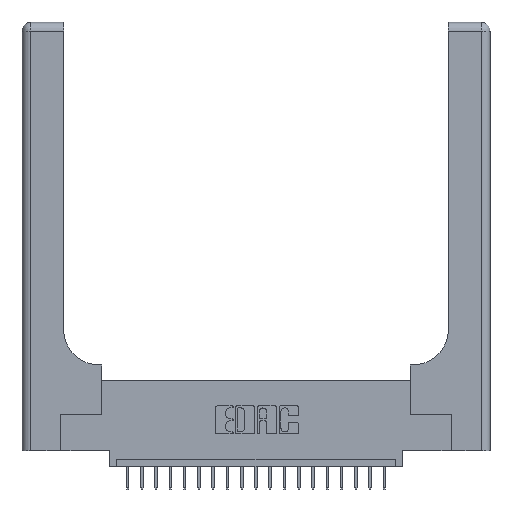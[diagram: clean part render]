
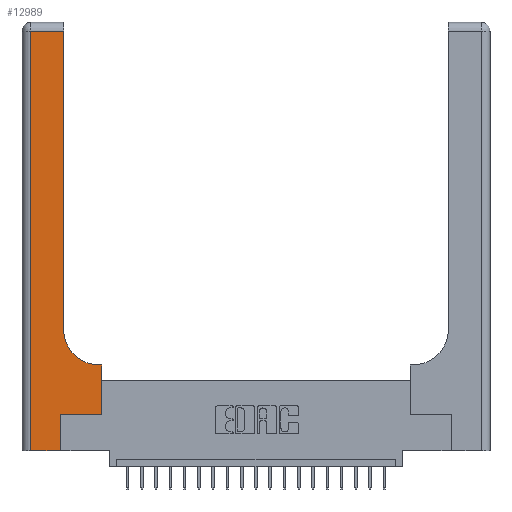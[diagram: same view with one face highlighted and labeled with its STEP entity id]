
A CAD part, top view. The second image highlights one B-rep face of the part: STEP entity #12989.
In plain terms, the highlighted planar face has unit normal (0, 0, 1).
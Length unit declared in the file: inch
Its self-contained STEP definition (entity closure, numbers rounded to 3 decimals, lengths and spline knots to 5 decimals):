
#396 = CARTESIAN_POINT ( 'NONE',  ( 0., 2.94, 0.37 ) ) ;
#868 = EDGE_CURVE ( 'NONE', #4343, #5429, #11607, .T. ) ;
#970 = CARTESIAN_POINT ( 'NONE',  ( 0.269, 0., 0.37 ) ) ;
#1243 = VERTEX_POINT ( 'NONE', #14700 ) ;
#1322 = CARTESIAN_POINT ( 'NONE',  ( 0.2915, 0.85, 0.37 ) ) ;
#1412 = DIRECTION ( 'NONE',  ( 1., 0., 0. ) ) ;
#2134 = DIRECTION ( 'NONE',  ( -1., 0., 0. ) ) ;
#2231 = CARTESIAN_POINT ( 'NONE',  ( 0.2915, 0.6, 0.37 ) ) ;
#2560 = EDGE_CURVE ( 'NONE', #10002, #20241, #6336, .T. ) ;
#2921 = ORIENTED_EDGE ( 'NONE', *, *, #21760, .T. ) ;
#3001 = EDGE_CURVE ( 'NONE', #5429, #19911, #18984, .T. ) ;
#3715 = DIRECTION ( 'NONE',  ( 0., 1., 0. ) ) ;
#4217 = ORIENTED_EDGE ( 'NONE', *, *, #19364, .T. ) ;
#4343 = VERTEX_POINT ( 'NONE', #16331 ) ;
#4400 = DIRECTION ( 'NONE',  ( 0., 1., 0. ) ) ;
#4521 = AXIS2_PLACEMENT_3D ( 'NONE', #8252, #11918, #1412 ) ;
#5310 = EDGE_CURVE ( 'NONE', #19329, #12533, #22745, .T. ) ;
#5429 = VERTEX_POINT ( 'NONE', #1322 ) ;
#5791 = LINE ( 'NONE', #2231, #21807 ) ;
#5943 = CARTESIAN_POINT ( 'NONE',  ( 0.2915, 3., 0.37 ) ) ;
#5963 = DIRECTION ( 'NONE',  ( -1., 0., 0. ) ) ;
#6336 = LINE ( 'NONE', #7860, #19887 ) ;
#7096 = PLANE ( 'NONE',  #11873 ) ;
#7426 = CARTESIAN_POINT ( 'NONE',  ( 0.5585, 0.25, 0.37 ) ) ;
#7774 = DIRECTION ( 'NONE',  ( 1., 0., 0. ) ) ;
#7860 = CARTESIAN_POINT ( 'NONE',  ( 0.5585, 0.25, 0.37 ) ) ;
#8252 = CARTESIAN_POINT ( 'NONE',  ( 0.5415, 0.85, 0.37 ) ) ;
#8469 = ORIENTED_EDGE ( 'NONE', *, *, #14919, .T. ) ;
#8563 = ORIENTED_EDGE ( 'NONE', *, *, #868, .T. ) ;
#8573 = CARTESIAN_POINT ( 'NONE',  ( 0.06, 3., 0.37 ) ) ;
#9168 = VECTOR ( 'NONE', #7774, 39.37008 ) ;
#10002 = VERTEX_POINT ( 'NONE', #7426 ) ;
#10135 = DIRECTION ( 'NONE',  ( 1., 0., 0. ) ) ;
#10136 = ORIENTED_EDGE ( 'NONE', *, *, #12586, .T. ) ;
#11075 = CARTESIAN_POINT ( 'NONE',  ( 0.269, 0.25, 0.37 ) ) ;
#11607 = CIRCLE ( 'NONE', #4521, 0.25 ) ;
#11807 = VECTOR ( 'NONE', #3715, 39.37008 ) ;
#11873 = AXIS2_PLACEMENT_3D ( 'NONE', #12497, #12250, #15935 ) ;
#11918 = DIRECTION ( 'NONE',  ( 0., 0., -1. ) ) ;
#11985 = CARTESIAN_POINT ( 'NONE',  ( 0., 0., 0.37 ) ) ;
#12163 = VECTOR ( 'NONE', #10135, 39.37008 ) ;
#12184 = DIRECTION ( 'NONE',  ( 0., -1., 0. ) ) ;
#12250 = DIRECTION ( 'NONE',  ( 0., 0., -1. ) ) ;
#12497 = CARTESIAN_POINT ( 'NONE',  ( 0., 3., 0.37 ) ) ;
#12533 = VERTEX_POINT ( 'NONE', #14290 ) ;
#12537 = CARTESIAN_POINT ( 'NONE',  ( 0.5585, 0.6, 0.37 ) ) ;
#12586 = EDGE_CURVE ( 'NONE', #19911, #19329, #14155, .T. ) ;
#12989 = ADVANCED_FACE ( 'NONE', ( #15210 ), #7096, .F. ) ;
#13323 = ORIENTED_EDGE ( 'NONE', *, *, #5310, .T. ) ;
#14065 = EDGE_LOOP ( 'NONE', ( #19680, #10136, #13323, #4217, #8469, #2921, #15923, #19437, #8563 ) ) ;
#14155 = LINE ( 'NONE', #396, #18546 ) ;
#14290 = CARTESIAN_POINT ( 'NONE',  ( 0.06, 0., 0.37 ) ) ;
#14700 = CARTESIAN_POINT ( 'NONE',  ( 0.269, 0., 0.37 ) ) ;
#14919 = EDGE_CURVE ( 'NONE', #1243, #20108, #20873, .T. ) ;
#15210 = FACE_OUTER_BOUND ( 'NONE', #14065, .T. ) ;
#15611 = VECTOR ( 'NONE', #20270, 39.37008 ) ;
#15923 = ORIENTED_EDGE ( 'NONE', *, *, #2560, .T. ) ;
#15935 = DIRECTION ( 'NONE',  ( -1., 0., 0. ) ) ;
#16331 = CARTESIAN_POINT ( 'NONE',  ( 0.5415, 0.6, 0.37 ) ) ;
#17223 = CARTESIAN_POINT ( 'NONE',  ( 0.06, 2.94, 0.37 ) ) ;
#18078 = VECTOR ( 'NONE', #12184, 39.37008 ) ;
#18546 = VECTOR ( 'NONE', #2134, 39.37008 ) ;
#18984 = LINE ( 'NONE', #5943, #11807 ) ;
#19329 = VERTEX_POINT ( 'NONE', #17223 ) ;
#19364 = EDGE_CURVE ( 'NONE', #12533, #1243, #21000, .T. ) ;
#19437 = ORIENTED_EDGE ( 'NONE', *, *, #20410, .T. ) ;
#19680 = ORIENTED_EDGE ( 'NONE', *, *, #3001, .T. ) ;
#19887 = VECTOR ( 'NONE', #4400, 39.37008 ) ;
#19911 = VERTEX_POINT ( 'NONE', #22182 ) ;
#20108 = VERTEX_POINT ( 'NONE', #22688 ) ;
#20241 = VERTEX_POINT ( 'NONE', #12537 ) ;
#20270 = DIRECTION ( 'NONE',  ( 0., 1., 0. ) ) ;
#20410 = EDGE_CURVE ( 'NONE', #20241, #4343, #5791, .T. ) ;
#20873 = LINE ( 'NONE', #970, #15611 ) ;
#21000 = LINE ( 'NONE', #11985, #12163 ) ;
#21010 = LINE ( 'NONE', #11075, #9168 ) ;
#21760 = EDGE_CURVE ( 'NONE', #20108, #10002, #21010, .T. ) ;
#21807 = VECTOR ( 'NONE', #5963, 39.37008 ) ;
#22182 = CARTESIAN_POINT ( 'NONE',  ( 0.2915, 2.94, 0.37 ) ) ;
#22688 = CARTESIAN_POINT ( 'NONE',  ( 0.269, 0.25, 0.37 ) ) ;
#22745 = LINE ( 'NONE', #8573, #18078 ) ;
